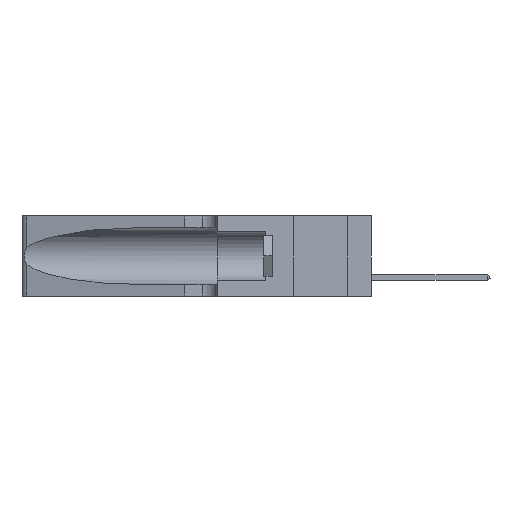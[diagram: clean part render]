
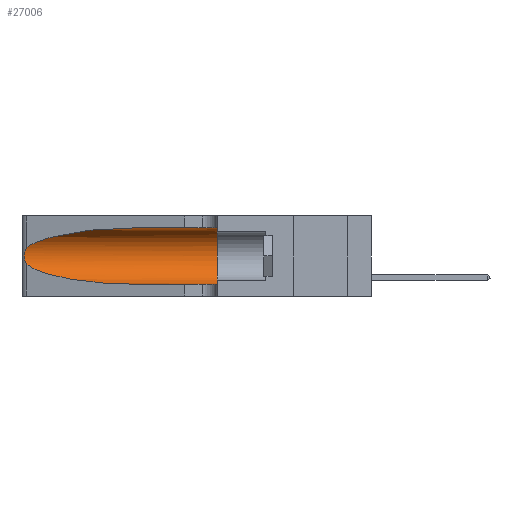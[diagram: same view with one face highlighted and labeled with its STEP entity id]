
A CAD part, left-side view. The second image highlights one B-rep face of the part: STEP entity #27006.
In plain terms, the highlighted cylindrical face has radius 3.308 mm (diameter 6.617 mm), a partial arc.
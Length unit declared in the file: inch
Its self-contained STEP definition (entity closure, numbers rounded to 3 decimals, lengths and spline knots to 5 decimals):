
#1251 = CARTESIAN_POINT ( 'NONE',  ( 0.25787, 1.23484, 0.2124 ) ) ;
#1356 = EDGE_CURVE ( 'NONE', #33122, #40927, #40965, .T. ) ;
#1629 = CARTESIAN_POINT ( 'NONE',  ( 0.1305, 0.72297, 0.05475 ) ) ;
#3401 = CARTESIAN_POINT ( 'NONE',  ( 0.1305, 0.35, 0.31525 ) ) ;
#5226 = CARTESIAN_POINT ( 'NONE',  ( 0.1305, 0.72297, 0.31525 ) ) ;
#6027 = CARTESIAN_POINT ( 'NONE',  ( 0.2373, 1.15595, 0.08982 ) ) ;
#7972 = CARTESIAN_POINT ( 'NONE',  ( 0.25487, 1.22718, 0.22369 ) ) ;
#8258 = CARTESIAN_POINT ( 'NONE',  ( 0.26075, 1.23896, 0.19203 ) ) ;
#8730 = LINE ( 'NONE', #33328, #28009 ) ;
#8749 =( BOUNDED_CURVE ( )  B_SPLINE_CURVE ( 3, ( #26545, #6027, #40405, #34613 ),
 .UNSPECIFIED., .F., .F. ) 
 B_SPLINE_CURVE_WITH_KNOTS ( ( 4, 4 ),
 ( 3.44316, 4.71239 ),
 .UNSPECIFIED. ) 
 CURVE ( )  GEOMETRIC_REPRESENTATION_ITEM ( )  RATIONAL_B_SPLINE_CURVE ( ( 1., 0.87, 0.87, 1. ) ) 
 REPRESENTATION_ITEM ( '' )  );
#9440 = VERTEX_POINT ( 'NONE', #1629 ) ;
#9815 = DIRECTION ( 'NONE',  ( 0., -1., 0. ) ) ;
#10739 = DIRECTION ( 'NONE',  ( 0., 0., -1. ) ) ;
#11260 = CARTESIAN_POINT ( 'NONE',  ( 0.25789, 1.23486, 0.15765 ) ) ;
#11745 = ORIENTED_EDGE ( 'NONE', *, *, #18980, .F. ) ;
#12604 = CYLINDRICAL_SURFACE ( 'NONE', #32236, 0.13025 ) ;
#14418 = AXIS2_PLACEMENT_3D ( 'NONE', #23064, #30094, #33720 ) ;
#14838 = CARTESIAN_POINT ( 'NONE',  ( 0.1305, 1.61858, 0.05475 ) ) ;
#14964 = CARTESIAN_POINT ( 'NONE',  ( 0.25555, 1.22994, 0.2215 ) ) ;
#15103 = CARTESIAN_POINT ( 'NONE',  ( 0.25487, 1.22718, 0.14631 ) ) ;
#15264 = CARTESIAN_POINT ( 'NONE',  ( 0.26075, 1.23896, 0.178 ) ) ;
#16110 = EDGE_LOOP ( 'NONE', ( #23413, #35699, #44053, #43434, #21774, #11745 ) ) ;
#16257 = VERTEX_POINT ( 'NONE', #38404 ) ;
#16564 = CARTESIAN_POINT ( 'NONE',  ( 0.25487, 1.22718, 0.22369 ) ) ;
#17569 = EDGE_CURVE ( 'NONE', #25698, #16257, #23276, .T. ) ;
#18980 = EDGE_CURVE ( 'NONE', #33122, #25698, #8730, .T. ) ;
#19732 = CARTESIAN_POINT ( 'NONE',  ( 0.1305, 0.72297, 0.31525 ) ) ;
#19754 = EDGE_CURVE ( 'NONE', #9440, #16257, #20447, .T. ) ;
#20447 = LINE ( 'NONE', #14838, #28497 ) ;
#21587 = CARTESIAN_POINT ( 'NONE',  ( 0.25487, 1.22718, 0.14631 ) ) ;
#21774 = ORIENTED_EDGE ( 'NONE', *, *, #17569, .F. ) ;
#23064 = CARTESIAN_POINT ( 'NONE',  ( 0.1305, 0.35, 0.185 ) ) ;
#23276 = CIRCLE ( 'NONE', #14418, 0.13025 ) ;
#23413 = ORIENTED_EDGE ( 'NONE', *, *, #1356, .T. ) ;
#24098 = B_SPLINE_CURVE_WITH_KNOTS ( 'NONE', 3,
 ( #7972, #14964, #42161, #1251, #39014, #35236, #8258, #15264, #35539, #25030, #11260, #28465, #25329, #21587 ),
 .UNSPECIFIED., .F., .F.,
 ( 4, 2, 2, 2, 2, 2, 4 ),
 ( 0., 0.00027, 0.00053, 0.00107, 0.0016, 0.00187, 0.00214 ),
 .UNSPECIFIED. ) ;
#24362 = FACE_OUTER_BOUND ( 'NONE', #16110, .T. ) ;
#25030 = CARTESIAN_POINT ( 'NONE',  ( 0.25856, 1.23593, 0.16098 ) ) ;
#25329 = CARTESIAN_POINT ( 'NONE',  ( 0.25555, 1.22993, 0.14849 ) ) ;
#25698 = VERTEX_POINT ( 'NONE', #3401 ) ;
#26545 = CARTESIAN_POINT ( 'NONE',  ( 0.25487, 1.22718, 0.14631 ) ) ;
#27006 = ADVANCED_FACE ( 'NONE', ( #24362 ), #12604, .F. ) ;
#28009 = VECTOR ( 'NONE', #9815, 39.37008 ) ;
#28465 = CARTESIAN_POINT ( 'NONE',  ( 0.25639, 1.23186, 0.15144 ) ) ;
#28497 = VECTOR ( 'NONE', #32229, 39.37008 ) ;
#28734 = DIRECTION ( 'NONE',  ( 0., -1., 0. ) ) ;
#29174 = CARTESIAN_POINT ( 'NONE',  ( 0.25487, 1.22718, 0.22369 ) ) ;
#30094 = DIRECTION ( 'NONE',  ( 0., 1., 0. ) ) ;
#32229 = DIRECTION ( 'NONE',  ( 0., -1., 0. ) ) ;
#32236 = AXIS2_PLACEMENT_3D ( 'NONE', #42725, #28734, #10739 ) ;
#33122 = VERTEX_POINT ( 'NONE', #19732 ) ;
#33328 = CARTESIAN_POINT ( 'NONE',  ( 0.1305, 1.61858, 0.31525 ) ) ;
#33720 = DIRECTION ( 'NONE',  ( 0., 0., 1. ) ) ;
#34613 = CARTESIAN_POINT ( 'NONE',  ( 0.1305, 0.72297, 0.05475 ) ) ;
#35236 = CARTESIAN_POINT ( 'NONE',  ( 0.26018, 1.23835, 0.19895 ) ) ;
#35539 = CARTESIAN_POINT ( 'NONE',  ( 0.26017, 1.23833, 0.17102 ) ) ;
#35699 = ORIENTED_EDGE ( 'NONE', *, *, #44116, .T. ) ;
#36497 = CARTESIAN_POINT ( 'NONE',  ( 0.18966, 0.96281, 0.31525 ) ) ;
#36656 = VERTEX_POINT ( 'NONE', #15103 ) ;
#38404 = CARTESIAN_POINT ( 'NONE',  ( 0.1305, 0.35, 0.05475 ) ) ;
#39014 = CARTESIAN_POINT ( 'NONE',  ( 0.25854, 1.2359, 0.20912 ) ) ;
#39713 = CARTESIAN_POINT ( 'NONE',  ( 0.2373, 1.15595, 0.28018 ) ) ;
#40405 = CARTESIAN_POINT ( 'NONE',  ( 0.18966, 0.96281, 0.05475 ) ) ;
#40927 = VERTEX_POINT ( 'NONE', #16564 ) ;
#40965 =( BOUNDED_CURVE ( )  B_SPLINE_CURVE ( 3, ( #5226, #36497, #39713, #29174 ),
 .UNSPECIFIED., .F., .F. ) 
 B_SPLINE_CURVE_WITH_KNOTS ( ( 4, 4 ),
 ( 1.5708, 2.84003 ),
 .UNSPECIFIED. ) 
 CURVE ( )  GEOMETRIC_REPRESENTATION_ITEM ( )  RATIONAL_B_SPLINE_CURVE ( ( 1., 0.87, 0.87, 1. ) ) 
 REPRESENTATION_ITEM ( '' )  );
#41719 = EDGE_CURVE ( 'NONE', #36656, #9440, #8749, .T. ) ;
#42161 = CARTESIAN_POINT ( 'NONE',  ( 0.25639, 1.23184, 0.21858 ) ) ;
#42725 = CARTESIAN_POINT ( 'NONE',  ( 0.1305, 1.61858, 0.185 ) ) ;
#43434 = ORIENTED_EDGE ( 'NONE', *, *, #19754, .T. ) ;
#44053 = ORIENTED_EDGE ( 'NONE', *, *, #41719, .T. ) ;
#44116 = EDGE_CURVE ( 'NONE', #40927, #36656, #24098, .T. ) ;
